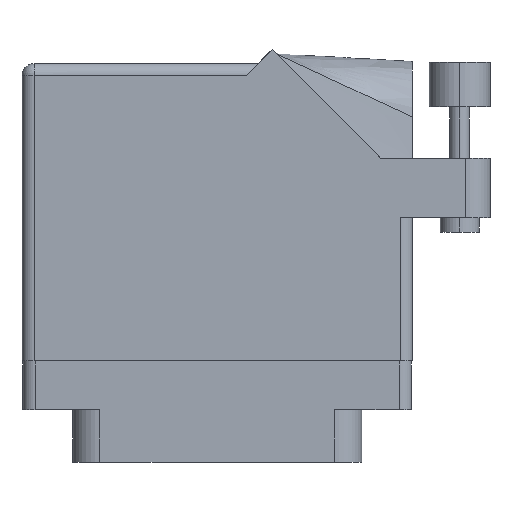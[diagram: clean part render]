
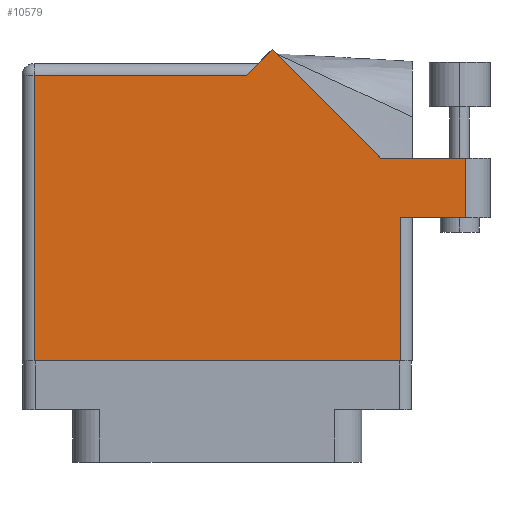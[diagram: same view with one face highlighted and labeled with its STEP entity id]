
A CAD part, front view. The second image highlights one B-rep face of the part: STEP entity #10579.
In plain terms, the highlighted face is planar.
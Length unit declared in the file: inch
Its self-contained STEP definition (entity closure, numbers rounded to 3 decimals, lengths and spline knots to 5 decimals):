
#532 = LINE ( 'NONE', #14065, #31948 ) ;
#1048 = LINE ( 'NONE', #19218, #26675 ) ;
#1428 = CARTESIAN_POINT ( 'NONE',  ( 0.28271, 1.50071, 0.455 ) ) ;
#1859 = CARTESIAN_POINT ( 'NONE',  ( 0.83942, 0.944, 0.455 ) ) ;
#1977 = DIRECTION ( 'NONE',  ( -1., 0., 0. ) ) ;
#3027 = CARTESIAN_POINT ( 'NONE',  ( -0.943, 1.368, 0.455 ) ) ;
#3047 = LINE ( 'NONE', #12492, #22066 ) ;
#3461 = ORIENTED_EDGE ( 'NONE', *, *, #27373, .T. ) ;
#4110 = EDGE_CURVE ( 'NONE', #30830, #18360, #27745, .T. ) ;
#4158 = VERTEX_POINT ( 'NONE', #3027 ) ;
#4860 = DIRECTION ( 'NONE',  ( -1., 0., 0. ) ) ;
#5403 = CARTESIAN_POINT ( 'NONE',  ( -1.005, 1.368, 0.455 ) ) ;
#6072 = VERTEX_POINT ( 'NONE', #20357 ) ;
#8844 = CARTESIAN_POINT ( 'NONE',  ( 1.28, 0.637, 0.455 ) ) ;
#10502 = DIRECTION ( 'NONE',  ( -1., 0., 0. ) ) ;
#10515 = CARTESIAN_POINT ( 'NONE',  ( 1.005, 0.637, 0.455 ) ) ;
#10579 = ADVANCED_FACE ( 'NONE', ( #26345 ), #22007, .F. ) ;
#12039 = EDGE_CURVE ( 'NONE', #12659, #30830, #23541, .T. ) ;
#12309 = ORIENTED_EDGE ( 'NONE', *, *, #24949, .T. ) ;
#12346 = CARTESIAN_POINT ( 'NONE',  ( -1.005, 1.43, 0.455 ) ) ;
#12384 = CARTESIAN_POINT ( 'NONE',  ( 0.943, -0.1, 0.455 ) ) ;
#12492 = CARTESIAN_POINT ( 'NONE',  ( 1.28, 0.944, 0.455 ) ) ;
#12659 = VERTEX_POINT ( 'NONE', #12384 ) ;
#13027 = DIRECTION ( 'NONE',  ( 1., 0., 0. ) ) ;
#13649 = VERTEX_POINT ( 'NONE', #1428 ) ;
#14065 = CARTESIAN_POINT ( 'NONE',  ( -0.943, -0.1, 0.455 ) ) ;
#14491 = VERTEX_POINT ( 'NONE', #28389 ) ;
#15675 = LINE ( 'NONE', #18835, #31571 ) ;
#15909 = VECTOR ( 'NONE', #10502, 39.37008 ) ;
#15998 = ORIENTED_EDGE ( 'NONE', *, *, #12039, .T. ) ;
#16387 = LINE ( 'NONE', #17135, #28832 ) ;
#16489 = ORIENTED_EDGE ( 'NONE', *, *, #17926, .T. ) ;
#17101 = EDGE_LOOP ( 'NONE', ( #27028, #28205, #12309, #31443, #31532, #3461, #31488, #16489, #15998 ) ) ;
#17135 = CARTESIAN_POINT ( 'NONE',  ( 1.405, 0.944, 0.455 ) ) ;
#17378 = CARTESIAN_POINT ( 'NONE',  ( -0.943, -0.1, 0.455 ) ) ;
#17505 = AXIS2_PLACEMENT_3D ( 'NONE', #12346, #27086, #4860 ) ;
#17654 = VECTOR ( 'NONE', #13027, 39.37008 ) ;
#17880 = EDGE_CURVE ( 'NONE', #4158, #24078, #532, .T. ) ;
#17926 = EDGE_CURVE ( 'NONE', #24078, #12659, #22689, .T. ) ;
#18360 = VERTEX_POINT ( 'NONE', #8844 ) ;
#18835 = CARTESIAN_POINT ( 'NONE',  ( 0.83942, 0.944, 0.455 ) ) ;
#19218 = CARTESIAN_POINT ( 'NONE',  ( 0.212, 1.43, 0.455 ) ) ;
#19544 = VECTOR ( 'NONE', #30922, 39.37008 ) ;
#19627 = VECTOR ( 'NONE', #30914, 39.37008 ) ;
#20357 = CARTESIAN_POINT ( 'NONE',  ( 0.15, 1.368, 0.455 ) ) ;
#21124 = CARTESIAN_POINT ( 'NONE',  ( -1.005, -0.1, 0.455 ) ) ;
#21506 = DIRECTION ( 'NONE',  ( -0.707, -0.707, 0. ) ) ;
#22007 = PLANE ( 'NONE',  #17505 ) ;
#22066 = VECTOR ( 'NONE', #28371, 39.37008 ) ;
#22147 = EDGE_CURVE ( 'NONE', #18360, #14491, #3047, .T. ) ;
#22531 = LINE ( 'NONE', #5403, #15909 ) ;
#22689 = LINE ( 'NONE', #21124, #19544 ) ;
#22815 = EDGE_CURVE ( 'NONE', #13649, #6072, #1048, .T. ) ;
#23541 = LINE ( 'NONE', #25812, #19627 ) ;
#24078 = VERTEX_POINT ( 'NONE', #17378 ) ;
#24869 = VERTEX_POINT ( 'NONE', #1859 ) ;
#24949 = EDGE_CURVE ( 'NONE', #14491, #24869, #16387, .T. ) ;
#25812 = CARTESIAN_POINT ( 'NONE',  ( 0.943, 0.637, 0.455 ) ) ;
#26307 = CARTESIAN_POINT ( 'NONE',  ( 0.943, 0.637, 0.455 ) ) ;
#26345 = FACE_OUTER_BOUND ( 'NONE', #17101, .T. ) ;
#26528 = DIRECTION ( 'NONE',  ( -0.707, 0.707, 0. ) ) ;
#26675 = VECTOR ( 'NONE', #21506, 39.37008 ) ;
#27028 = ORIENTED_EDGE ( 'NONE', *, *, #4110, .T. ) ;
#27086 = DIRECTION ( 'NONE',  ( 0., 0., -1. ) ) ;
#27373 = EDGE_CURVE ( 'NONE', #6072, #4158, #22531, .T. ) ;
#27745 = LINE ( 'NONE', #10515, #17654 ) ;
#28205 = ORIENTED_EDGE ( 'NONE', *, *, #22147, .T. ) ;
#28371 = DIRECTION ( 'NONE',  ( 0., 1., 0. ) ) ;
#28389 = CARTESIAN_POINT ( 'NONE',  ( 1.28, 0.944, 0.455 ) ) ;
#28602 = DIRECTION ( 'NONE',  ( 0., -1., 0. ) ) ;
#28832 = VECTOR ( 'NONE', #1977, 39.37008 ) ;
#30816 = EDGE_CURVE ( 'NONE', #24869, #13649, #15675, .T. ) ;
#30830 = VERTEX_POINT ( 'NONE', #26307 ) ;
#30914 = DIRECTION ( 'NONE',  ( 0., 1., 0. ) ) ;
#30922 = DIRECTION ( 'NONE',  ( 1., 0., 0. ) ) ;
#31443 = ORIENTED_EDGE ( 'NONE', *, *, #30816, .T. ) ;
#31488 = ORIENTED_EDGE ( 'NONE', *, *, #17880, .T. ) ;
#31532 = ORIENTED_EDGE ( 'NONE', *, *, #22815, .T. ) ;
#31571 = VECTOR ( 'NONE', #26528, 39.37008 ) ;
#31948 = VECTOR ( 'NONE', #28602, 39.37008 ) ;
